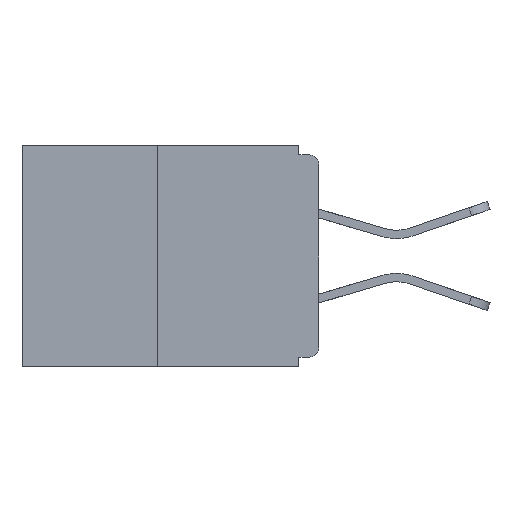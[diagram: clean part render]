
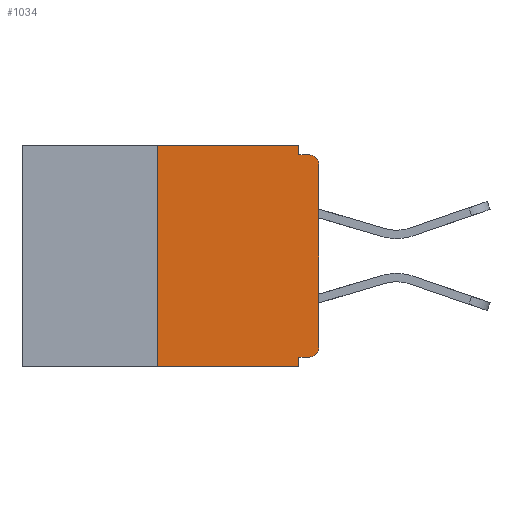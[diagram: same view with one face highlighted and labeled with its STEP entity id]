
A CAD part, left-side view. The second image highlights one B-rep face of the part: STEP entity #1034.
In plain terms, the highlighted planar face has unit normal (-1, 0, 0).
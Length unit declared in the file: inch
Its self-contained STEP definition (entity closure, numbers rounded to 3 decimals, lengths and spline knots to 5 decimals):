
#87 = ORIENTED_EDGE ( 'NONE', *, *, #3573, .T. ) ;
#401 = VERTEX_POINT ( 'NONE', #5278 ) ;
#610 = VECTOR ( 'NONE', #4959, 39.37008 ) ;
#1034 = ADVANCED_FACE ( 'NONE', ( #7211 ), #12383, .F. ) ;
#1121 = CARTESIAN_POINT ( 'NONE',  ( 0., 0.25, -0.343 ) ) ;
#1129 = LINE ( 'NONE', #4677, #14919 ) ;
#1193 = CARTESIAN_POINT ( 'NONE',  ( 0., 0.031, 0. ) ) ;
#1272 = ORIENTED_EDGE ( 'NONE', *, *, #8561, .F. ) ;
#1509 = CARTESIAN_POINT ( 'NONE',  ( 0., 0.015, -0.313 ) ) ;
#1510 = CARTESIAN_POINT ( 'NONE',  ( 0., 0., -0.015 ) ) ;
#1517 = VERTEX_POINT ( 'NONE', #15624 ) ;
#2212 = DIRECTION ( 'NONE',  ( 1., 0., 0. ) ) ;
#2466 = VECTOR ( 'NONE', #10735, 39.37008 ) ;
#2519 = VECTOR ( 'NONE', #12773, 39.37008 ) ;
#2622 = AXIS2_PLACEMENT_3D ( 'NONE', #16257, #2212, #15132 ) ;
#2665 = VECTOR ( 'NONE', #16290, 39.37008 ) ;
#3312 = CARTESIAN_POINT ( 'NONE',  ( 0., 0.015, -0.03 ) ) ;
#3573 = EDGE_CURVE ( 'NONE', #13167, #401, #14553, .T. ) ;
#3850 = CARTESIAN_POINT ( 'NONE',  ( 0., 0., -0.03 ) ) ;
#3953 = DIRECTION ( 'NONE',  ( 0., -1., 0. ) ) ;
#4009 = ORIENTED_EDGE ( 'NONE', *, *, #10531, .F. ) ;
#4157 = CARTESIAN_POINT ( 'NONE',  ( 0., 0.031, -0.015 ) ) ;
#4207 = CARTESIAN_POINT ( 'NONE',  ( 0., 0.015, -0.328 ) ) ;
#4215 = DIRECTION ( 'NONE',  ( 0., 0., -1. ) ) ;
#4530 = VECTOR ( 'NONE', #3953, 39.37008 ) ;
#4557 = LINE ( 'NONE', #12916, #14386 ) ;
#4570 = DIRECTION ( 'NONE',  ( 0., 0., -1. ) ) ;
#4638 = AXIS2_PLACEMENT_3D ( 'NONE', #1509, #6632, #4215 ) ;
#4677 = CARTESIAN_POINT ( 'NONE',  ( 0., 0.46, 0. ) ) ;
#4959 = DIRECTION ( 'NONE',  ( 0., 0., -1. ) ) ;
#5015 = ORIENTED_EDGE ( 'NONE', *, *, #7320, .F. ) ;
#5095 = CARTESIAN_POINT ( 'NONE',  ( 0., 0.031, 0. ) ) ;
#5278 = CARTESIAN_POINT ( 'NONE',  ( 0., 0., -0.313 ) ) ;
#6025 = VERTEX_POINT ( 'NONE', #3850 ) ;
#6105 = DIRECTION ( 'NONE',  ( 0., -1., 0. ) ) ;
#6147 = AXIS2_PLACEMENT_3D ( 'NONE', #3312, #12242, #4570 ) ;
#6577 = DIRECTION ( 'NONE',  ( 0., 0., 1. ) ) ;
#6631 = LINE ( 'NONE', #9739, #2665 ) ;
#6632 = DIRECTION ( 'NONE',  ( -1., 0., 0. ) ) ;
#7082 = CARTESIAN_POINT ( 'NONE',  ( 0., 0.46, -0.343 ) ) ;
#7211 = FACE_OUTER_BOUND ( 'NONE', #11489, .T. ) ;
#7320 = EDGE_CURVE ( 'NONE', #11202, #15863, #8249, .T. ) ;
#7394 = CARTESIAN_POINT ( 'NONE',  ( 0., 0.031, -0.343 ) ) ;
#7482 = LINE ( 'NONE', #5095, #2519 ) ;
#7585 = VECTOR ( 'NONE', #14759, 39.37008 ) ;
#7931 = LINE ( 'NONE', #1510, #4530 ) ;
#8143 = VERTEX_POINT ( 'NONE', #1193 ) ;
#8147 = ORIENTED_EDGE ( 'NONE', *, *, #11173, .T. ) ;
#8249 = LINE ( 'NONE', #9530, #2466 ) ;
#8519 = ORIENTED_EDGE ( 'NONE', *, *, #13780, .F. ) ;
#8558 = EDGE_CURVE ( 'NONE', #401, #6025, #4557, .T. ) ;
#8561 = EDGE_CURVE ( 'NONE', #12589, #1517, #7931, .T. ) ;
#9530 = CARTESIAN_POINT ( 'NONE',  ( 0., 0.25, 0. ) ) ;
#9739 = CARTESIAN_POINT ( 'NONE',  ( 0., 0., -0.328 ) ) ;
#9747 = EDGE_CURVE ( 'NONE', #15863, #8143, #1129, .T. ) ;
#9802 = LINE ( 'NONE', #7082, #7585 ) ;
#10302 = CARTESIAN_POINT ( 'NONE',  ( 0., 0.031, -0.343 ) ) ;
#10497 = VERTEX_POINT ( 'NONE', #10302 ) ;
#10531 = EDGE_CURVE ( 'NONE', #8143, #12589, #7482, .T. ) ;
#10735 = DIRECTION ( 'NONE',  ( 0., 0., 1. ) ) ;
#11173 = EDGE_CURVE ( 'NONE', #6025, #1517, #11708, .T. ) ;
#11202 = VERTEX_POINT ( 'NONE', #1121 ) ;
#11351 = ORIENTED_EDGE ( 'NONE', *, *, #9747, .F. ) ;
#11487 = ORIENTED_EDGE ( 'NONE', *, *, #14839, .F. ) ;
#11489 = EDGE_LOOP ( 'NONE', ( #11351, #5015, #14779, #8519, #11487, #87, #13526, #8147, #1272, #4009 ) ) ;
#11708 = CIRCLE ( 'NONE', #6147, 0.015 ) ;
#12242 = DIRECTION ( 'NONE',  ( -1., 0., 0. ) ) ;
#12383 = PLANE ( 'NONE',  #2622 ) ;
#12589 = VERTEX_POINT ( 'NONE', #4157 ) ;
#12646 = CARTESIAN_POINT ( 'NONE',  ( 0., 0.031, -0.328 ) ) ;
#12773 = DIRECTION ( 'NONE',  ( 0., 0., -1. ) ) ;
#12916 = CARTESIAN_POINT ( 'NONE',  ( 0., 0., 0. ) ) ;
#13167 = VERTEX_POINT ( 'NONE', #4207 ) ;
#13208 = LINE ( 'NONE', #7394, #610 ) ;
#13526 = ORIENTED_EDGE ( 'NONE', *, *, #8558, .T. ) ;
#13596 = EDGE_CURVE ( 'NONE', #11202, #10497, #9802, .T. ) ;
#13780 = EDGE_CURVE ( 'NONE', #14894, #10497, #13208, .T. ) ;
#14386 = VECTOR ( 'NONE', #6577, 39.37008 ) ;
#14553 = CIRCLE ( 'NONE', #4638, 0.015 ) ;
#14759 = DIRECTION ( 'NONE',  ( 0., -1., 0. ) ) ;
#14779 = ORIENTED_EDGE ( 'NONE', *, *, #13596, .T. ) ;
#14839 = EDGE_CURVE ( 'NONE', #13167, #14894, #6631, .T. ) ;
#14876 = CARTESIAN_POINT ( 'NONE',  ( 0., 0.25, 0. ) ) ;
#14894 = VERTEX_POINT ( 'NONE', #12646 ) ;
#14919 = VECTOR ( 'NONE', #6105, 39.37008 ) ;
#15132 = DIRECTION ( 'NONE',  ( 0., 0., -1. ) ) ;
#15624 = CARTESIAN_POINT ( 'NONE',  ( 0., 0.015, -0.015 ) ) ;
#15863 = VERTEX_POINT ( 'NONE', #14876 ) ;
#16257 = CARTESIAN_POINT ( 'NONE',  ( 0., 0.46, 0. ) ) ;
#16290 = DIRECTION ( 'NONE',  ( 0., 1., 0. ) ) ;
